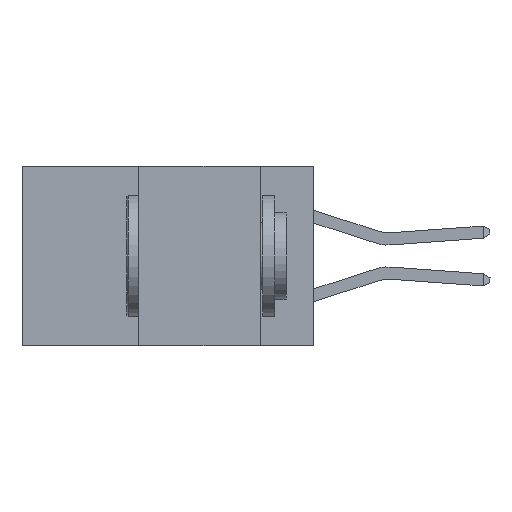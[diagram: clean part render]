
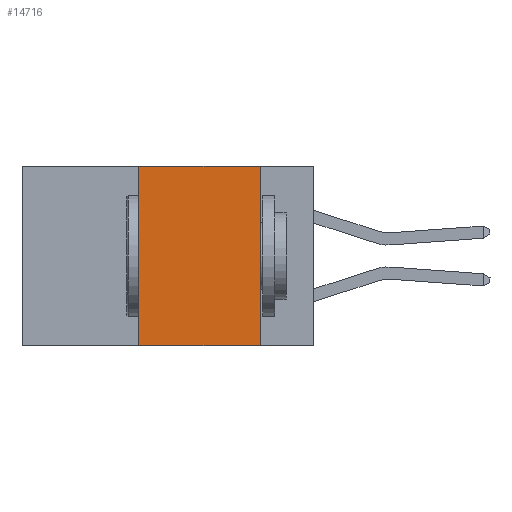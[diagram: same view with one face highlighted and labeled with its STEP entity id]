
A CAD part, left-side view. The second image highlights one B-rep face of the part: STEP entity #14716.
In plain terms, the highlighted planar face has unit normal (-1, 0, 0).
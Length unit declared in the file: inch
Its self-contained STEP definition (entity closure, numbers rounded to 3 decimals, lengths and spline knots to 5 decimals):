
#485 = VERTEX_POINT ( 'NONE', #4755 ) ;
#884 = LINE ( 'NONE', #4558, #8520 ) ;
#1217 = DIRECTION ( 'NONE',  ( 0., 0., -1. ) ) ;
#1363 = LINE ( 'NONE', #14131, #5888 ) ;
#2140 = FACE_OUTER_BOUND ( 'NONE', #17163, .T. ) ;
#2846 = LINE ( 'NONE', #18499, #5421 ) ;
#2884 = EDGE_CURVE ( 'NONE', #485, #16784, #884, .T. ) ;
#3299 = EDGE_CURVE ( 'NONE', #485, #4173, #1363, .T. ) ;
#3783 = DIRECTION ( 'NONE',  ( 0., 0., 1. ) ) ;
#4071 = ORIENTED_EDGE ( 'NONE', *, *, #2884, .F. ) ;
#4173 = VERTEX_POINT ( 'NONE', #16720 ) ;
#4376 = ORIENTED_EDGE ( 'NONE', *, *, #14968, .F. ) ;
#4558 = CARTESIAN_POINT ( 'NONE',  ( 0., 0.36, 0. ) ) ;
#4607 = DIRECTION ( 'NONE',  ( 0., -1., 0. ) ) ;
#4755 = CARTESIAN_POINT ( 'NONE',  ( 0., 0.36, -0.37 ) ) ;
#5231 = ORIENTED_EDGE ( 'NONE', *, *, #8578, .F. ) ;
#5421 = VECTOR ( 'NONE', #12660, 39.37008 ) ;
#5888 = VECTOR ( 'NONE', #19148, 39.37008 ) ;
#6833 = VECTOR ( 'NONE', #4607, 39.37008 ) ;
#8210 = ORIENTED_EDGE ( 'NONE', *, *, #3299, .T. ) ;
#8520 = VECTOR ( 'NONE', #3783, 39.37008 ) ;
#8578 = EDGE_CURVE ( 'NONE', #16784, #18412, #14940, .T. ) ;
#10322 = DIRECTION ( 'NONE',  ( 1., 0., 0. ) ) ;
#12187 = CARTESIAN_POINT ( 'NONE',  ( 0., 0.6, 0. ) ) ;
#12660 = DIRECTION ( 'NONE',  ( 0., 0., -1. ) ) ;
#14131 = CARTESIAN_POINT ( 'NONE',  ( 0., 0.6, -0.37 ) ) ;
#14716 = ADVANCED_FACE ( 'NONE', ( #2140 ), #17748, .F. ) ;
#14940 = LINE ( 'NONE', #12187, #6833 ) ;
#14968 = EDGE_CURVE ( 'NONE', #18412, #4173, #2846, .T. ) ;
#15144 = CARTESIAN_POINT ( 'NONE',  ( 0., 0.36, 0. ) ) ;
#15480 = AXIS2_PLACEMENT_3D ( 'NONE', #19221, #10322, #1217 ) ;
#16590 = CARTESIAN_POINT ( 'NONE',  ( 0., 0.11, 0. ) ) ;
#16720 = CARTESIAN_POINT ( 'NONE',  ( 0., 0.11, -0.37 ) ) ;
#16784 = VERTEX_POINT ( 'NONE', #15144 ) ;
#17163 = EDGE_LOOP ( 'NONE', ( #4376, #5231, #4071, #8210 ) ) ;
#17748 = PLANE ( 'NONE',  #15480 ) ;
#18412 = VERTEX_POINT ( 'NONE', #16590 ) ;
#18499 = CARTESIAN_POINT ( 'NONE',  ( 0., 0.11, 0. ) ) ;
#19148 = DIRECTION ( 'NONE',  ( 0., -1., 0. ) ) ;
#19221 = CARTESIAN_POINT ( 'NONE',  ( 0., 0.6, 0. ) ) ;
